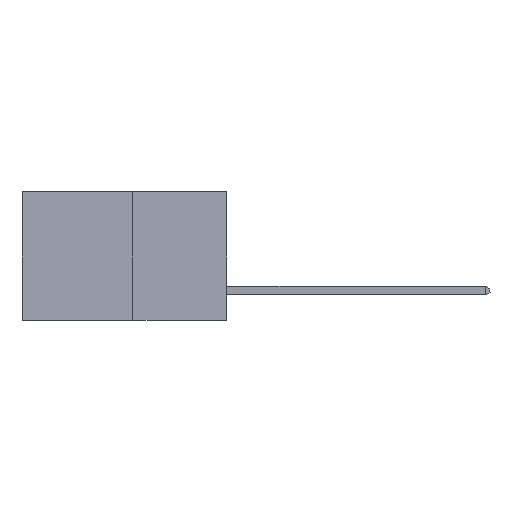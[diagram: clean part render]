
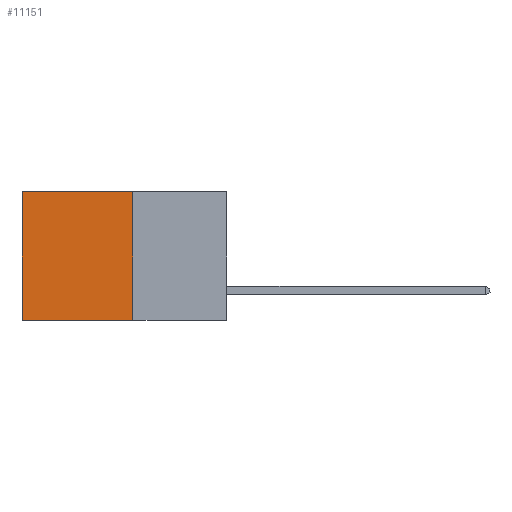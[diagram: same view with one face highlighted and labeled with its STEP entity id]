
A CAD part, left-side view. The second image highlights one B-rep face of the part: STEP entity #11151.
In plain terms, the highlighted planar face has unit normal (-1, 0, 0).
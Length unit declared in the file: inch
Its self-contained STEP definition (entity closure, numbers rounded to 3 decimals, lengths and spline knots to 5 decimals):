
#442 = DIRECTION ( 'NONE',  ( 0., 1., 0. ) ) ;
#1111 = ORIENTED_EDGE ( 'NONE', *, *, #3142, .F. ) ;
#1139 = DIRECTION ( 'NONE',  ( 0., 0., -1. ) ) ;
#1462 = VECTOR ( 'NONE', #5825, 39.37008 ) ;
#1894 = EDGE_CURVE ( 'NONE', #4679, #12935, #13227, .T. ) ;
#2351 = VERTEX_POINT ( 'NONE', #10046 ) ;
#2653 = ORIENTED_EDGE ( 'NONE', *, *, #6610, .T. ) ;
#2661 = LINE ( 'NONE', #14120, #8542 ) ;
#3142 = EDGE_CURVE ( 'NONE', #2351, #4679, #12113, .T. ) ;
#3367 = EDGE_CURVE ( 'NONE', #2351, #13641, #10071, .T. ) ;
#3400 = DIRECTION ( 'NONE',  ( 0., 0., -1. ) ) ;
#4679 = VERTEX_POINT ( 'NONE', #14142 ) ;
#5825 = DIRECTION ( 'NONE',  ( 0., 1., 0. ) ) ;
#5844 = EDGE_LOOP ( 'NONE', ( #2653, #9603, #1111, #8837 ) ) ;
#6141 = CARTESIAN_POINT ( 'NONE',  ( 0.277, 0.27, -0.37 ) ) ;
#6361 = CARTESIAN_POINT ( 'NONE',  ( 0.277, 0.59, 0. ) ) ;
#6610 = EDGE_CURVE ( 'NONE', #13641, #12935, #2661, .T. ) ;
#8317 = DIRECTION ( 'NONE',  ( 1., 0., 0. ) ) ;
#8542 = VECTOR ( 'NONE', #3400, 39.37008 ) ;
#8837 = ORIENTED_EDGE ( 'NONE', *, *, #3367, .T. ) ;
#9138 = VECTOR ( 'NONE', #13327, 39.37008 ) ;
#9603 = ORIENTED_EDGE ( 'NONE', *, *, #1894, .F. ) ;
#9768 = VECTOR ( 'NONE', #442, 39.37008 ) ;
#9862 = CARTESIAN_POINT ( 'NONE',  ( 0.277, 0.27, 0. ) ) ;
#10046 = CARTESIAN_POINT ( 'NONE',  ( 0.277, 0.27, 0. ) ) ;
#10071 = LINE ( 'NONE', #9862, #9768 ) ;
#10999 = FACE_OUTER_BOUND ( 'NONE', #5844, .T. ) ;
#11151 = ADVANCED_FACE ( 'NONE', ( #10999 ), #14257, .F. ) ;
#11735 = CARTESIAN_POINT ( 'NONE',  ( 0.277, 0.59, -0.37 ) ) ;
#12113 = LINE ( 'NONE', #12339, #9138 ) ;
#12339 = CARTESIAN_POINT ( 'NONE',  ( 0.277, 0.27, -0.37 ) ) ;
#12935 = VERTEX_POINT ( 'NONE', #11735 ) ;
#13227 = LINE ( 'NONE', #6141, #1462 ) ;
#13315 = CARTESIAN_POINT ( 'NONE',  ( 0.277, 0.27, -0.37 ) ) ;
#13327 = DIRECTION ( 'NONE',  ( 0., 0., -1. ) ) ;
#13641 = VERTEX_POINT ( 'NONE', #6361 ) ;
#13780 = AXIS2_PLACEMENT_3D ( 'NONE', #13315, #8317, #1139 ) ;
#14120 = CARTESIAN_POINT ( 'NONE',  ( 0.277, 0.59, -0.37 ) ) ;
#14142 = CARTESIAN_POINT ( 'NONE',  ( 0.277, 0.27, -0.37 ) ) ;
#14257 = PLANE ( 'NONE',  #13780 ) ;
